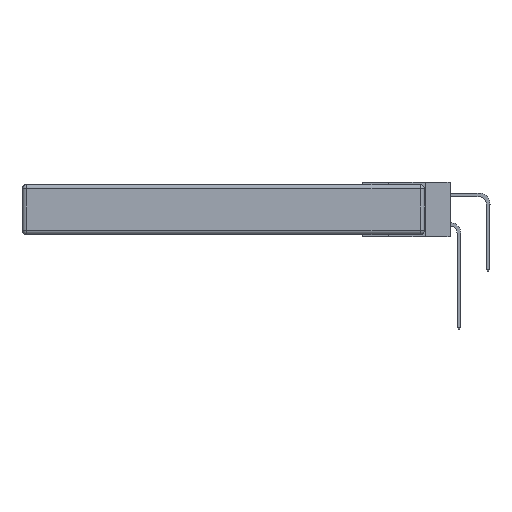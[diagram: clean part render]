
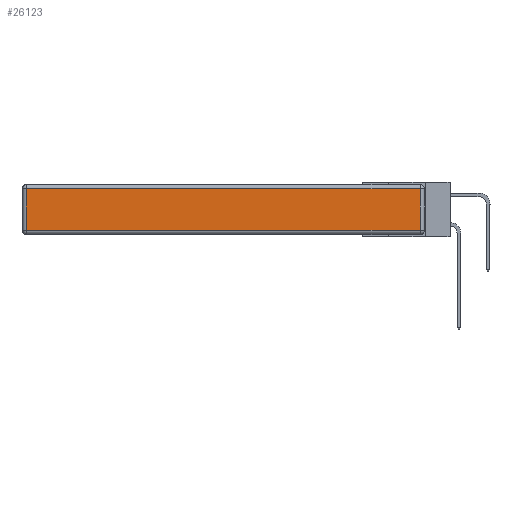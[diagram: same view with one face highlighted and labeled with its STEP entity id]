
A CAD part, left-side view. The second image highlights one B-rep face of the part: STEP entity #26123.
In plain terms, the highlighted planar face has unit normal (-1, 0, 0).
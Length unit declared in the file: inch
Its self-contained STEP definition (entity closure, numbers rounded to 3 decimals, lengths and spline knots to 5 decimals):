
#481 = CARTESIAN_POINT ( 'NONE',  ( 0., 0., -0.343 ) ) ;
#2072 = ORIENTED_EDGE ( 'NONE', *, *, #29189, .T. ) ;
#2570 = CARTESIAN_POINT ( 'NONE',  ( 0., 0.03, -0.03 ) ) ;
#2951 = LINE ( 'NONE', #13887, #3392 ) ;
#3392 = VECTOR ( 'NONE', #27965, 39.37008 ) ;
#3416 = CARTESIAN_POINT ( 'NONE',  ( 0., 2.72, -0.03 ) ) ;
#6487 = LINE ( 'NONE', #14274, #27027 ) ;
#6578 = DIRECTION ( 'NONE',  ( 0., -1., 0. ) ) ;
#6964 = DIRECTION ( 'NONE',  ( 0., 0., -1. ) ) ;
#7422 = LINE ( 'NONE', #33545, #32203 ) ;
#7724 = VERTEX_POINT ( 'NONE', #25692 ) ;
#8071 = FACE_OUTER_BOUND ( 'NONE', #16111, .T. ) ;
#8784 = PLANE ( 'NONE',  #28445 ) ;
#10795 = VERTEX_POINT ( 'NONE', #3416 ) ;
#11836 = ORIENTED_EDGE ( 'NONE', *, *, #20702, .T. ) ;
#12354 = VERTEX_POINT ( 'NONE', #26000 ) ;
#13887 = CARTESIAN_POINT ( 'NONE',  ( 0., 2.75, -0.03 ) ) ;
#14274 = CARTESIAN_POINT ( 'NONE',  ( 0., 0.03, -0.343 ) ) ;
#14933 = ORIENTED_EDGE ( 'NONE', *, *, #31845, .T. ) ;
#16111 = EDGE_LOOP ( 'NONE', ( #2072, #14933, #17008, #11836 ) ) ;
#17008 = ORIENTED_EDGE ( 'NONE', *, *, #21509, .T. ) ;
#17009 = DIRECTION ( 'NONE',  ( 0., 0., 1. ) ) ;
#19235 = DIRECTION ( 'NONE',  ( -1., 0., 0. ) ) ;
#20702 = EDGE_CURVE ( 'NONE', #10795, #7724, #27206, .T. ) ;
#21509 = EDGE_CURVE ( 'NONE', #24006, #10795, #2951, .T. ) ;
#22673 = CARTESIAN_POINT ( 'NONE',  ( 0., 2.72, -0.343 ) ) ;
#24006 = VERTEX_POINT ( 'NONE', #2570 ) ;
#25692 = CARTESIAN_POINT ( 'NONE',  ( 0., 2.72, -0.313 ) ) ;
#26000 = CARTESIAN_POINT ( 'NONE',  ( 0., 0.03, -0.313 ) ) ;
#26123 = ADVANCED_FACE ( 'NONE', ( #8071 ), #8784, .T. ) ;
#27027 = VECTOR ( 'NONE', #33052, 39.37008 ) ;
#27206 = LINE ( 'NONE', #22673, #31015 ) ;
#27965 = DIRECTION ( 'NONE',  ( 0., 1., 0. ) ) ;
#28445 = AXIS2_PLACEMENT_3D ( 'NONE', #481, #19235, #17009 ) ;
#29189 = EDGE_CURVE ( 'NONE', #7724, #12354, #7422, .T. ) ;
#31015 = VECTOR ( 'NONE', #6964, 39.37008 ) ;
#31845 = EDGE_CURVE ( 'NONE', #12354, #24006, #6487, .T. ) ;
#32203 = VECTOR ( 'NONE', #6578, 39.37008 ) ;
#33052 = DIRECTION ( 'NONE',  ( 0., 0., 1. ) ) ;
#33545 = CARTESIAN_POINT ( 'NONE',  ( 0., 0., -0.313 ) ) ;
